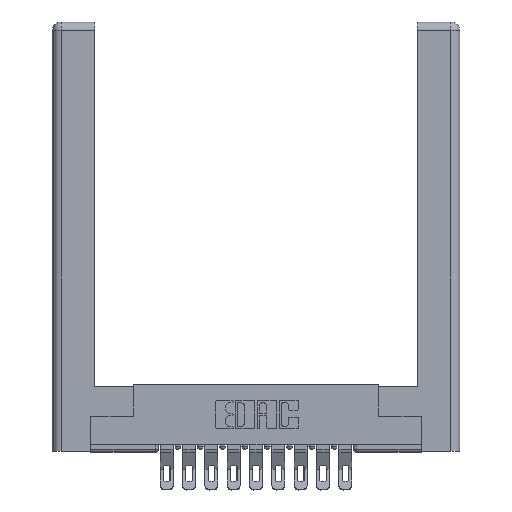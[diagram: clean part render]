
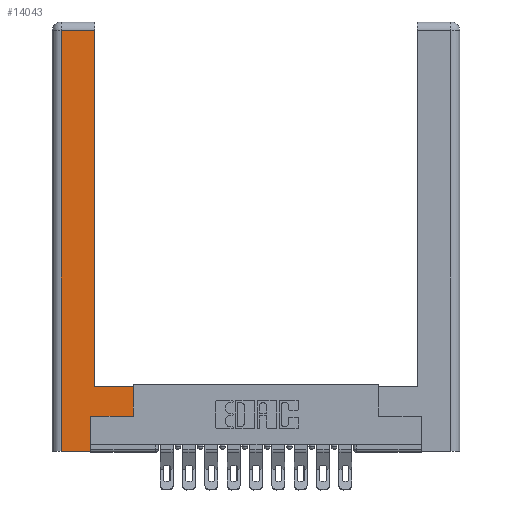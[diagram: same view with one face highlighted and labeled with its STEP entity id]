
A CAD part, top view. The second image highlights one B-rep face of the part: STEP entity #14043.
In plain terms, the highlighted planar face has unit normal (0, 0, 1).
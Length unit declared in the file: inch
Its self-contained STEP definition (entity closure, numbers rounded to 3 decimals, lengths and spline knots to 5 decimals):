
#171 = VECTOR ( 'NONE', #2587, 39.37008 ) ;
#172 = CARTESIAN_POINT ( 'NONE',  ( 0.295, 3., 0. ) ) ;
#182 = CARTESIAN_POINT ( 'NONE',  ( 0.295, 0.45, 0. ) ) ;
#194 = DIRECTION ( 'NONE',  ( 1., 0., 0. ) ) ;
#278 = CARTESIAN_POINT ( 'NONE',  ( 0.265, 0.245, 0. ) ) ;
#679 = CARTESIAN_POINT ( 'NONE',  ( 0.265, 0., 0. ) ) ;
#2106 = CARTESIAN_POINT ( 'NONE',  ( 0.0615, 0., 0. ) ) ;
#2162 = VERTEX_POINT ( 'NONE', #11386 ) ;
#2374 = EDGE_CURVE ( 'NONE', #2162, #4296, #9748, .T. ) ;
#2546 = EDGE_CURVE ( 'NONE', #4444, #13151, #4064, .T. ) ;
#2587 = DIRECTION ( 'NONE',  ( 0., 1., 0. ) ) ;
#3259 = DIRECTION ( 'NONE',  ( 0., 0., -1. ) ) ;
#3346 = CARTESIAN_POINT ( 'NONE',  ( 0.565, 0.45, 0. ) ) ;
#3370 = CARTESIAN_POINT ( 'NONE',  ( 0.0615, 2.94, 0. ) ) ;
#3689 = VECTOR ( 'NONE', #14700, 39.37008 ) ;
#4064 = LINE ( 'NONE', #11951, #171 ) ;
#4194 = CARTESIAN_POINT ( 'NONE',  ( 0.565, 0.245, 0. ) ) ;
#4216 = FACE_OUTER_BOUND ( 'NONE', #9055, .T. ) ;
#4296 = VERTEX_POINT ( 'NONE', #13381 ) ;
#4444 = VERTEX_POINT ( 'NONE', #679 ) ;
#4525 = DIRECTION ( 'NONE',  ( 0., 1., 0. ) ) ;
#5613 = DIRECTION ( 'NONE',  ( 0., -1., 0. ) ) ;
#5715 = ORIENTED_EDGE ( 'NONE', *, *, #13070, .T. ) ;
#5807 = EDGE_CURVE ( 'NONE', #14029, #7606, #15122, .T. ) ;
#6109 = DIRECTION ( 'NONE',  ( -1., 0., 0. ) ) ;
#6544 = DIRECTION ( 'NONE',  ( -1., 0., 0. ) ) ;
#6829 = ORIENTED_EDGE ( 'NONE', *, *, #13086, .T. ) ;
#7606 = VERTEX_POINT ( 'NONE', #9237 ) ;
#7653 = CARTESIAN_POINT ( 'NONE',  ( 0.295, 2.94, 0. ) ) ;
#7822 = EDGE_CURVE ( 'NONE', #7606, #4444, #8235, .T. ) ;
#8228 = VECTOR ( 'NONE', #6544, 39.37008 ) ;
#8235 = LINE ( 'NONE', #13133, #13590 ) ;
#8597 = VECTOR ( 'NONE', #11918, 39.37008 ) ;
#8625 = VERTEX_POINT ( 'NONE', #12469 ) ;
#8689 = ORIENTED_EDGE ( 'NONE', *, *, #2374, .T. ) ;
#8717 = LINE ( 'NONE', #3346, #10615 ) ;
#9055 = EDGE_LOOP ( 'NONE', ( #11594, #5715, #14568, #11163, #9062, #6829, #12141, #8689 ) ) ;
#9062 = ORIENTED_EDGE ( 'NONE', *, *, #2546, .T. ) ;
#9237 = CARTESIAN_POINT ( 'NONE',  ( 0.0615, 0., 0. ) ) ;
#9418 = VECTOR ( 'NONE', #5613, 39.37008 ) ;
#9748 = LINE ( 'NONE', #182, #12118 ) ;
#10092 = EDGE_CURVE ( 'NONE', #8625, #2162, #8717, .T. ) ;
#10391 = CARTESIAN_POINT ( 'NONE',  ( 0., 0., 0. ) ) ;
#10440 = DIRECTION ( 'NONE',  ( -1., 0., 0. ) ) ;
#10615 = VECTOR ( 'NONE', #4525, 39.37008 ) ;
#11163 = ORIENTED_EDGE ( 'NONE', *, *, #7822, .T. ) ;
#11386 = CARTESIAN_POINT ( 'NONE',  ( 0.565, 0.45, 0. ) ) ;
#11594 = ORIENTED_EDGE ( 'NONE', *, *, #12892, .T. ) ;
#11903 = LINE ( 'NONE', #172, #8597 ) ;
#11918 = DIRECTION ( 'NONE',  ( 0., 1., 0. ) ) ;
#11951 = CARTESIAN_POINT ( 'NONE',  ( 0.265, 0.245, 0. ) ) ;
#12033 = AXIS2_PLACEMENT_3D ( 'NONE', #10391, #3259, #10440 ) ;
#12118 = VECTOR ( 'NONE', #6109, 39.37008 ) ;
#12141 = ORIENTED_EDGE ( 'NONE', *, *, #10092, .T. ) ;
#12279 = LINE ( 'NONE', #13571, #8228 ) ;
#12469 = CARTESIAN_POINT ( 'NONE',  ( 0.565, 0.245, 0. ) ) ;
#12726 = PLANE ( 'NONE',  #12033 ) ;
#12892 = EDGE_CURVE ( 'NONE', #4296, #13095, #11903, .T. ) ;
#13070 = EDGE_CURVE ( 'NONE', #13095, #14029, #12279, .T. ) ;
#13086 = EDGE_CURVE ( 'NONE', #13151, #8625, #14863, .T. ) ;
#13095 = VERTEX_POINT ( 'NONE', #7653 ) ;
#13133 = CARTESIAN_POINT ( 'NONE',  ( 0.265, 0., 0. ) ) ;
#13151 = VERTEX_POINT ( 'NONE', #278 ) ;
#13381 = CARTESIAN_POINT ( 'NONE',  ( 0.295, 0.45, 0. ) ) ;
#13571 = CARTESIAN_POINT ( 'NONE',  ( 0.0615, 2.94, 0. ) ) ;
#13590 = VECTOR ( 'NONE', #194, 39.37008 ) ;
#14029 = VERTEX_POINT ( 'NONE', #3370 ) ;
#14043 = ADVANCED_FACE ( 'NONE', ( #4216 ), #12726, .F. ) ;
#14568 = ORIENTED_EDGE ( 'NONE', *, *, #5807, .T. ) ;
#14700 = DIRECTION ( 'NONE',  ( 1., 0., 0. ) ) ;
#14863 = LINE ( 'NONE', #4194, #3689 ) ;
#15122 = LINE ( 'NONE', #2106, #9418 ) ;
